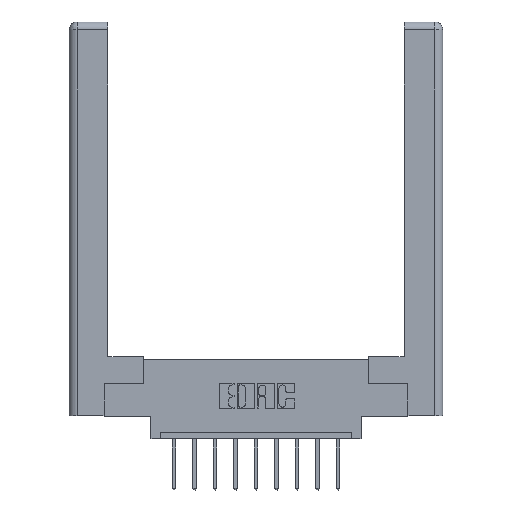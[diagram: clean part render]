
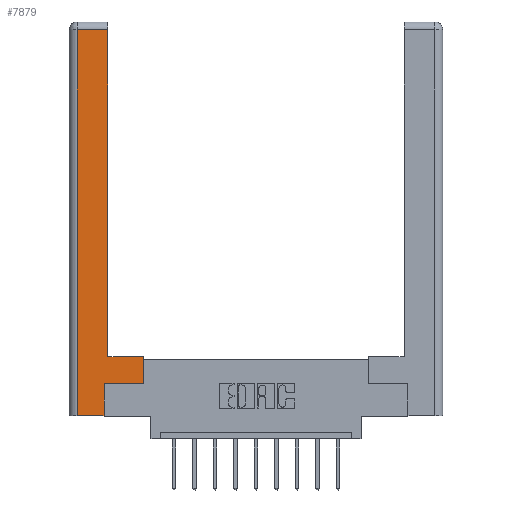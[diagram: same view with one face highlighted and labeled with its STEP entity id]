
A CAD part, top view. The second image highlights one B-rep face of the part: STEP entity #7879.
In plain terms, the highlighted planar face has unit normal (0, 0, 1).
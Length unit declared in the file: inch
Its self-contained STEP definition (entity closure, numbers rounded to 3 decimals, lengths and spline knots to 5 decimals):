
#62 = VECTOR ( 'NONE', #1522, 39.37008 ) ;
#577 = VERTEX_POINT ( 'NONE', #9208 ) ;
#612 = VECTOR ( 'NONE', #5582, 39.37008 ) ;
#811 = AXIS2_PLACEMENT_3D ( 'NONE', #2239, #9652, #8660 ) ;
#973 = LINE ( 'NONE', #8550, #1324 ) ;
#1177 = EDGE_CURVE ( 'NONE', #13565, #577, #11783, .T. ) ;
#1324 = VECTOR ( 'NONE', #8464, 39.37008 ) ;
#1511 = VERTEX_POINT ( 'NONE', #11148 ) ;
#1522 = DIRECTION ( 'NONE',  ( 1., 0., 0. ) ) ;
#1811 = CARTESIAN_POINT ( 'NONE',  ( 0.565, 0.245, 0. ) ) ;
#1903 = VERTEX_POINT ( 'NONE', #11927 ) ;
#1953 = VERTEX_POINT ( 'NONE', #3416 ) ;
#2239 = CARTESIAN_POINT ( 'NONE',  ( 0., 0., 0. ) ) ;
#2875 = EDGE_CURVE ( 'NONE', #1953, #7723, #3763, .T. ) ;
#2971 = CARTESIAN_POINT ( 'NONE',  ( 0.265, 0., 0. ) ) ;
#3416 = CARTESIAN_POINT ( 'NONE',  ( 0.295, 2.94, 0. ) ) ;
#3490 = VERTEX_POINT ( 'NONE', #9589 ) ;
#3574 = ORIENTED_EDGE ( 'NONE', *, *, #2875, .T. ) ;
#3763 = LINE ( 'NONE', #12488, #7402 ) ;
#3775 = EDGE_CURVE ( 'NONE', #1511, #13565, #12672, .T. ) ;
#3972 = ORIENTED_EDGE ( 'NONE', *, *, #3775, .T. ) ;
#4422 = ORIENTED_EDGE ( 'NONE', *, *, #8379, .T. ) ;
#4549 = PLANE ( 'NONE',  #811 ) ;
#4789 = ORIENTED_EDGE ( 'NONE', *, *, #5059, .T. ) ;
#4851 = CARTESIAN_POINT ( 'NONE',  ( 0.565, 0.245, 0. ) ) ;
#4914 = VECTOR ( 'NONE', #5123, 39.37008 ) ;
#4977 = DIRECTION ( 'NONE',  ( -1., 0., 0. ) ) ;
#5059 = EDGE_CURVE ( 'NONE', #7723, #1903, #7782, .T. ) ;
#5123 = DIRECTION ( 'NONE',  ( 1., 0., 0. ) ) ;
#5322 = CARTESIAN_POINT ( 'NONE',  ( 0.265, 0.245, 0. ) ) ;
#5469 = LINE ( 'NONE', #5322, #13270 ) ;
#5582 = DIRECTION ( 'NONE',  ( 0., -1., 0. ) ) ;
#5746 = DIRECTION ( 'NONE',  ( 0., 1., 0. ) ) ;
#6754 = ORIENTED_EDGE ( 'NONE', *, *, #1177, .T. ) ;
#6943 = LINE ( 'NONE', #7881, #13243 ) ;
#7122 = CARTESIAN_POINT ( 'NONE',  ( 0.0615, 2.94, 0. ) ) ;
#7173 = ORIENTED_EDGE ( 'NONE', *, *, #11066, .T. ) ;
#7237 = CARTESIAN_POINT ( 'NONE',  ( 0.295, 0.45, 0. ) ) ;
#7378 = EDGE_CURVE ( 'NONE', #8915, #1953, #6943, .T. ) ;
#7402 = VECTOR ( 'NONE', #4977, 39.37008 ) ;
#7723 = VERTEX_POINT ( 'NONE', #7122 ) ;
#7782 = LINE ( 'NONE', #11049, #612 ) ;
#7879 = ADVANCED_FACE ( 'NONE', ( #8730 ), #4549, .F. ) ;
#7881 = CARTESIAN_POINT ( 'NONE',  ( 0.295, 3., 0. ) ) ;
#8373 = LINE ( 'NONE', #2971, #4914 ) ;
#8379 = EDGE_CURVE ( 'NONE', #1903, #3490, #8373, .T. ) ;
#8464 = DIRECTION ( 'NONE',  ( -1., 0., 0. ) ) ;
#8550 = CARTESIAN_POINT ( 'NONE',  ( 0.295, 0.45, 0. ) ) ;
#8660 = DIRECTION ( 'NONE',  ( -1., 0., 0. ) ) ;
#8730 = FACE_OUTER_BOUND ( 'NONE', #9997, .T. ) ;
#8915 = VERTEX_POINT ( 'NONE', #7237 ) ;
#9208 = CARTESIAN_POINT ( 'NONE',  ( 0.565, 0.45, 0. ) ) ;
#9589 = CARTESIAN_POINT ( 'NONE',  ( 0.265, 0., 0. ) ) ;
#9652 = DIRECTION ( 'NONE',  ( 0., 0., -1. ) ) ;
#9997 = EDGE_LOOP ( 'NONE', ( #13697, #3574, #4789, #4422, #7173, #3972, #6754, #11195 ) ) ;
#10099 = VECTOR ( 'NONE', #5746, 39.37008 ) ;
#10505 = EDGE_CURVE ( 'NONE', #577, #8915, #973, .T. ) ;
#10627 = DIRECTION ( 'NONE',  ( 0., 1., 0. ) ) ;
#11049 = CARTESIAN_POINT ( 'NONE',  ( 0.0615, 0., 0. ) ) ;
#11066 = EDGE_CURVE ( 'NONE', #3490, #1511, #5469, .T. ) ;
#11070 = DIRECTION ( 'NONE',  ( 0., 1., 0. ) ) ;
#11148 = CARTESIAN_POINT ( 'NONE',  ( 0.265, 0.245, 0. ) ) ;
#11195 = ORIENTED_EDGE ( 'NONE', *, *, #10505, .T. ) ;
#11783 = LINE ( 'NONE', #13069, #10099 ) ;
#11927 = CARTESIAN_POINT ( 'NONE',  ( 0.0615, 0., 0. ) ) ;
#12488 = CARTESIAN_POINT ( 'NONE',  ( 0.0615, 2.94, 0. ) ) ;
#12672 = LINE ( 'NONE', #4851, #62 ) ;
#13069 = CARTESIAN_POINT ( 'NONE',  ( 0.565, 0.45, 0. ) ) ;
#13243 = VECTOR ( 'NONE', #11070, 39.37008 ) ;
#13270 = VECTOR ( 'NONE', #10627, 39.37008 ) ;
#13565 = VERTEX_POINT ( 'NONE', #1811 ) ;
#13697 = ORIENTED_EDGE ( 'NONE', *, *, #7378, .T. ) ;
